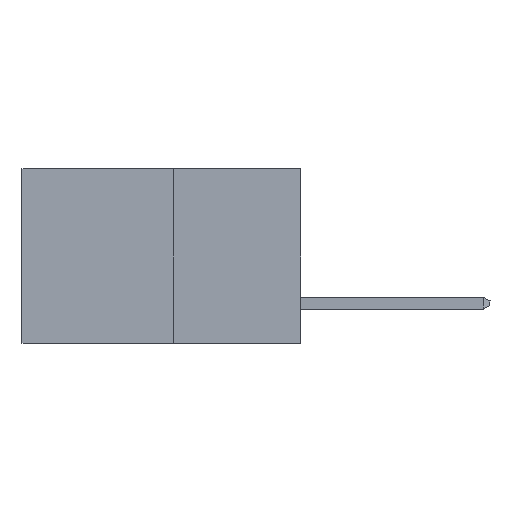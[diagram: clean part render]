
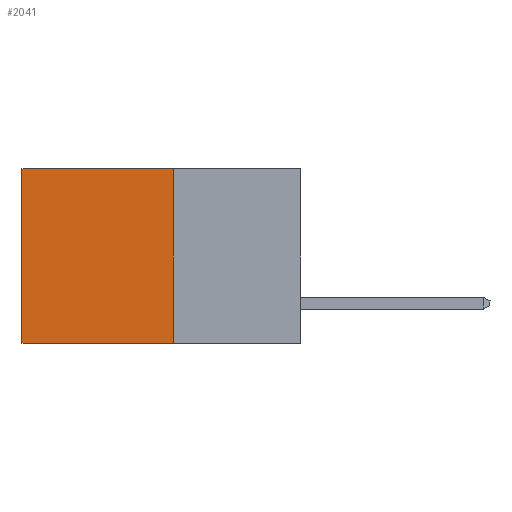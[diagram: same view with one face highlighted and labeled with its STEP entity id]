
A CAD part, left-side view. The second image highlights one B-rep face of the part: STEP entity #2041.
In plain terms, the highlighted planar face has unit normal (-1, 0, 0).
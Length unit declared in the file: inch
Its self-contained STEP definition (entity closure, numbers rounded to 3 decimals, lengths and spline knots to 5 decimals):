
#93 = VECTOR ( 'NONE', #2691, 39.37008 ) ;
#461 = LINE ( 'NONE', #4212, #7249 ) ;
#548 = VECTOR ( 'NONE', #4914, 39.37008 ) ;
#737 = LINE ( 'NONE', #1039, #3894 ) ;
#896 = ORIENTED_EDGE ( 'NONE', *, *, #7051, .T. ) ;
#972 = ORIENTED_EDGE ( 'NONE', *, *, #6641, .F. ) ;
#1039 = CARTESIAN_POINT ( 'NONE',  ( 0.277, 0.59, -0.37 ) ) ;
#1183 = DIRECTION ( 'NONE',  ( 0., 0., -1. ) ) ;
#1603 = ORIENTED_EDGE ( 'NONE', *, *, #7756, .T. ) ;
#1754 = LINE ( 'NONE', #2697, #93 ) ;
#1761 = DIRECTION ( 'NONE',  ( 0., 0., -1. ) ) ;
#2041 = ADVANCED_FACE ( 'NONE', ( #3956 ), #7457, .F. ) ;
#2691 = DIRECTION ( 'NONE',  ( 0., 1., 0. ) ) ;
#2697 = CARTESIAN_POINT ( 'NONE',  ( 0.277, 0.27, 0. ) ) ;
#3860 = CARTESIAN_POINT ( 'NONE',  ( 0.277, 0.27, -0.37 ) ) ;
#3894 = VECTOR ( 'NONE', #1761, 39.37008 ) ;
#3956 = FACE_OUTER_BOUND ( 'NONE', #6200, .T. ) ;
#4109 = LINE ( 'NONE', #4906, #548 ) ;
#4141 = DIRECTION ( 'NONE',  ( 0., 0., -1. ) ) ;
#4173 = VERTEX_POINT ( 'NONE', #7476 ) ;
#4212 = CARTESIAN_POINT ( 'NONE',  ( 0.277, 0.27, -0.37 ) ) ;
#4325 = VERTEX_POINT ( 'NONE', #7387 ) ;
#4906 = CARTESIAN_POINT ( 'NONE',  ( 0.277, 0.27, -0.37 ) ) ;
#4914 = DIRECTION ( 'NONE',  ( 0., 1., 0. ) ) ;
#5557 = VERTEX_POINT ( 'NONE', #5572 ) ;
#5572 = CARTESIAN_POINT ( 'NONE',  ( 0.277, 0.59, -0.37 ) ) ;
#5640 = EDGE_CURVE ( 'NONE', #4325, #5657, #461, .T. ) ;
#5657 = VERTEX_POINT ( 'NONE', #3860 ) ;
#5920 = AXIS2_PLACEMENT_3D ( 'NONE', #6872, #7680, #1183 ) ;
#6200 = EDGE_LOOP ( 'NONE', ( #1603, #972, #6428, #896 ) ) ;
#6428 = ORIENTED_EDGE ( 'NONE', *, *, #5640, .F. ) ;
#6641 = EDGE_CURVE ( 'NONE', #5657, #5557, #4109, .T. ) ;
#6872 = CARTESIAN_POINT ( 'NONE',  ( 0.277, 0.27, -0.37 ) ) ;
#7051 = EDGE_CURVE ( 'NONE', #4325, #4173, #1754, .T. ) ;
#7249 = VECTOR ( 'NONE', #4141, 39.37008 ) ;
#7387 = CARTESIAN_POINT ( 'NONE',  ( 0.277, 0.27, 0. ) ) ;
#7457 = PLANE ( 'NONE',  #5920 ) ;
#7476 = CARTESIAN_POINT ( 'NONE',  ( 0.277, 0.59, 0. ) ) ;
#7680 = DIRECTION ( 'NONE',  ( 1., 0., 0. ) ) ;
#7756 = EDGE_CURVE ( 'NONE', #4173, #5557, #737, .T. ) ;
